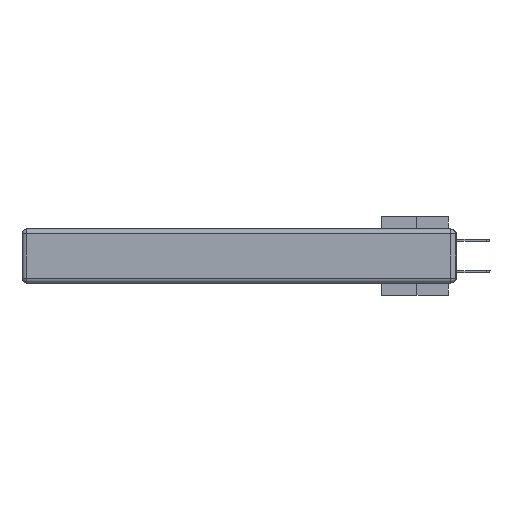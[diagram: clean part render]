
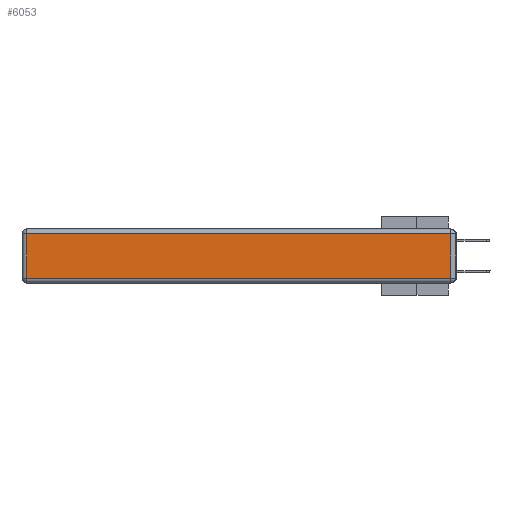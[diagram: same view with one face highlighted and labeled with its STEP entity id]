
A CAD part, left-side view. The second image highlights one B-rep face of the part: STEP entity #6053.
In plain terms, the highlighted planar face has unit normal (-1, 0, 0).
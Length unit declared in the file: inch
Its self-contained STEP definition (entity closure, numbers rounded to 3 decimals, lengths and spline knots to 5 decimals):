
#545 = ORIENTED_EDGE ( 'NONE', *, *, #6758, .T. ) ;
#1501 = LINE ( 'NONE', #5689, #5496 ) ;
#4887 = CARTESIAN_POINT ( 'NONE',  ( 0., 0., -0.313 ) ) ;
#5496 = VECTOR ( 'NONE', #11306, 39.37008 ) ;
#5689 = CARTESIAN_POINT ( 'NONE',  ( 0., 2.75, -0.03 ) ) ;
#6053 = ADVANCED_FACE ( 'NONE', ( #15381 ), #17850, .T. ) ;
#6274 = VERTEX_POINT ( 'NONE', #15841 ) ;
#6597 = DIRECTION ( 'NONE',  ( 0., 0., 1. ) ) ;
#6758 = EDGE_CURVE ( 'NONE', #35880, #6274, #1501, .T. ) ;
#8947 = VECTOR ( 'NONE', #22388, 39.37008 ) ;
#9472 = DIRECTION ( 'NONE',  ( -1., 0., 0. ) ) ;
#9576 = CARTESIAN_POINT ( 'NONE',  ( 0., 0.03, -0.03 ) ) ;
#10733 = LINE ( 'NONE', #15125, #29095 ) ;
#11306 = DIRECTION ( 'NONE',  ( 0., 1., 0. ) ) ;
#13641 = EDGE_CURVE ( 'NONE', #16985, #26656, #31783, .T. ) ;
#14923 = CARTESIAN_POINT ( 'NONE',  ( 0., 2.72, -0.343 ) ) ;
#15125 = CARTESIAN_POINT ( 'NONE',  ( 0., 0.03, -0.343 ) ) ;
#15381 = FACE_OUTER_BOUND ( 'NONE', #31310, .T. ) ;
#15841 = CARTESIAN_POINT ( 'NONE',  ( 0., 2.72, -0.03 ) ) ;
#16985 = VERTEX_POINT ( 'NONE', #27328 ) ;
#17212 = ORIENTED_EDGE ( 'NONE', *, *, #13641, .T. ) ;
#17850 = PLANE ( 'NONE',  #28772 ) ;
#20464 = EDGE_CURVE ( 'NONE', #6274, #16985, #21578, .T. ) ;
#20715 = CARTESIAN_POINT ( 'NONE',  ( 0., 0., -0.343 ) ) ;
#21578 = LINE ( 'NONE', #14923, #34583 ) ;
#21688 = EDGE_CURVE ( 'NONE', #26656, #35880, #10733, .T. ) ;
#22388 = DIRECTION ( 'NONE',  ( 0., -1., 0. ) ) ;
#23689 = DIRECTION ( 'NONE',  ( 0., 0., -1. ) ) ;
#26656 = VERTEX_POINT ( 'NONE', #33341 ) ;
#27328 = CARTESIAN_POINT ( 'NONE',  ( 0., 2.72, -0.313 ) ) ;
#28772 = AXIS2_PLACEMENT_3D ( 'NONE', #20715, #9472, #6597 ) ;
#29095 = VECTOR ( 'NONE', #29531, 39.37008 ) ;
#29531 = DIRECTION ( 'NONE',  ( 0., 0., 1. ) ) ;
#31310 = EDGE_LOOP ( 'NONE', ( #17212, #35526, #545, #36485 ) ) ;
#31783 = LINE ( 'NONE', #4887, #8947 ) ;
#33341 = CARTESIAN_POINT ( 'NONE',  ( 0., 0.03, -0.313 ) ) ;
#34583 = VECTOR ( 'NONE', #23689, 39.37008 ) ;
#35526 = ORIENTED_EDGE ( 'NONE', *, *, #21688, .T. ) ;
#35880 = VERTEX_POINT ( 'NONE', #9576 ) ;
#36485 = ORIENTED_EDGE ( 'NONE', *, *, #20464, .T. ) ;
